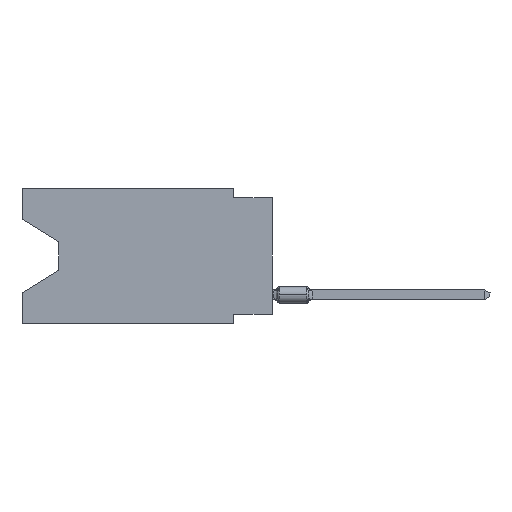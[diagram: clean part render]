
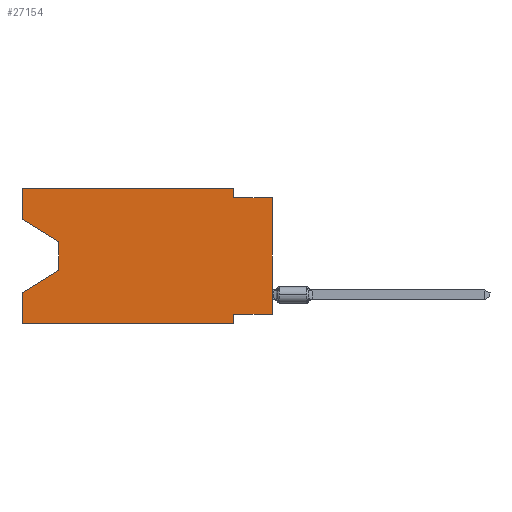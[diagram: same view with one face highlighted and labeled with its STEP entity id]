
A CAD part, left-side view. The second image highlights one B-rep face of the part: STEP entity #27154.
In plain terms, the highlighted planar face has unit normal (-1, 0, 0).
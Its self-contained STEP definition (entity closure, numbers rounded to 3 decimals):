
#526 = CARTESIAN_POINT ( 'NONE',  ( 0., 13.97, -3.505 ) ) ;
#664 = DIRECTION ( 'NONE',  ( 0., -1., 0. ) ) ;
#1069 = ORIENTED_EDGE ( 'NONE', *, *, #26090, .F. ) ;
#1391 = EDGE_LOOP ( 'NONE', ( #17667, #36850, #2581, #44364, #42576, #38319, #42074, #20796, #1069, #49209, #34071, #36737 ) ) ;
#1396 = VERTEX_POINT ( 'NONE', #10982 ) ;
#2026 = VECTOR ( 'NONE', #36965, 1000. ) ;
#2171 = EDGE_CURVE ( 'NONE', #13277, #44504, #7679, .T. ) ;
#2351 = VERTEX_POINT ( 'NONE', #28143 ) ;
#2581 = ORIENTED_EDGE ( 'NONE', *, *, #29722, .T. ) ;
#3048 = VECTOR ( 'NONE', #36815, 1000. ) ;
#4729 = VECTOR ( 'NONE', #34349, 1000. ) ;
#4867 = VECTOR ( 'NONE', #17695, 1000. ) ;
#5331 = EDGE_CURVE ( 'NONE', #1396, #10738, #50507, .T. ) ;
#6120 = CARTESIAN_POINT ( 'NONE',  ( 0., 13.97, -5.385 ) ) ;
#7053 = EDGE_CURVE ( 'NONE', #44504, #2351, #36006, .T. ) ;
#7087 = DIRECTION ( 'NONE',  ( 0., 0., -1. ) ) ;
#7679 = LINE ( 'NONE', #27627, #4729 ) ;
#8245 = LINE ( 'NONE', #28692, #2026 ) ;
#8286 = EDGE_CURVE ( 'NONE', #1396, #45997, #10141, .T. ) ;
#9231 = VECTOR ( 'NONE', #21283, 1000. ) ;
#9792 = AXIS2_PLACEMENT_3D ( 'NONE', #19267, #10950, #31141 ) ;
#10141 = LINE ( 'NONE', #45111, #4867 ) ;
#10183 = DIRECTION ( 'NONE',  ( 0., 0., 1. ) ) ;
#10738 = VERTEX_POINT ( 'NONE', #27488 ) ;
#10950 = DIRECTION ( 'NONE',  ( 1., 0., 0. ) ) ;
#10982 = CARTESIAN_POINT ( 'NONE',  ( 0., 0., -8.255 ) ) ;
#11155 = VECTOR ( 'NONE', #664, 1000. ) ;
#12522 = CARTESIAN_POINT ( 'NONE',  ( 0., 2.54, -8.89 ) ) ;
#13277 = VERTEX_POINT ( 'NONE', #42623 ) ;
#13744 = VERTEX_POINT ( 'NONE', #28295 ) ;
#14079 = VERTEX_POINT ( 'NONE', #526 ) ;
#14117 = CARTESIAN_POINT ( 'NONE',  ( 0., 16.383, -2.038 ) ) ;
#14336 = LINE ( 'NONE', #34513, #37570 ) ;
#14949 = VECTOR ( 'NONE', #44714, 1000. ) ;
#14989 = EDGE_CURVE ( 'NONE', #13277, #14079, #45178, .T. ) ;
#16276 = CARTESIAN_POINT ( 'NONE',  ( 0., 13.97, -5.385 ) ) ;
#16737 = EDGE_CURVE ( 'NONE', #2351, #28925, #19806, .T. ) ;
#17667 = ORIENTED_EDGE ( 'NONE', *, *, #14989, .T. ) ;
#17695 = DIRECTION ( 'NONE',  ( 0., 1., 0. ) ) ;
#19267 = CARTESIAN_POINT ( 'NONE',  ( 0., 16.383, 0. ) ) ;
#19806 = LINE ( 'NONE', #35804, #40992 ) ;
#20115 = CARTESIAN_POINT ( 'NONE',  ( 0., 16.383, -8.89 ) ) ;
#20515 = VERTEX_POINT ( 'NONE', #6120 ) ;
#20796 = ORIENTED_EDGE ( 'NONE', *, *, #5331, .T. ) ;
#21283 = DIRECTION ( 'NONE',  ( 0., -1., 0. ) ) ;
#22308 = EDGE_CURVE ( 'NONE', #13744, #24663, #43385, .T. ) ;
#23673 = DIRECTION ( 'NONE',  ( 0., 0., -1. ) ) ;
#24663 = VERTEX_POINT ( 'NONE', #12522 ) ;
#26090 = EDGE_CURVE ( 'NONE', #28925, #10738, #40700, .T. ) ;
#26498 = PLANE ( 'NONE',  #9792 ) ;
#27154 = ADVANCED_FACE ( 'NONE', ( #35022 ), #26498, .F. ) ;
#27488 = CARTESIAN_POINT ( 'NONE',  ( 0., 0., -0.635 ) ) ;
#27627 = CARTESIAN_POINT ( 'NONE',  ( 0., 16.383, 0. ) ) ;
#28143 = CARTESIAN_POINT ( 'NONE',  ( 0., 2.54, 0. ) ) ;
#28295 = CARTESIAN_POINT ( 'NONE',  ( 0., 16.383, -8.89 ) ) ;
#28692 = CARTESIAN_POINT ( 'NONE',  ( 0., 2.54, -8.89 ) ) ;
#28896 = DIRECTION ( 'NONE',  ( 0., -0.855, -0.519 ) ) ;
#28925 = VERTEX_POINT ( 'NONE', #33757 ) ;
#28927 = LINE ( 'NONE', #16276, #14949 ) ;
#29060 = CARTESIAN_POINT ( 'NONE',  ( 0., 0., -0.635 ) ) ;
#29722 = EDGE_CURVE ( 'NONE', #20515, #32320, #28927, .T. ) ;
#30378 = CARTESIAN_POINT ( 'NONE',  ( 0., 2.54, -8.255 ) ) ;
#30651 = LINE ( 'NONE', #42552, #49188 ) ;
#31141 = DIRECTION ( 'NONE',  ( 0., 0., -1. ) ) ;
#32320 = VERTEX_POINT ( 'NONE', #46088 ) ;
#33757 = CARTESIAN_POINT ( 'NONE',  ( 0., 2.54, -0.635 ) ) ;
#34011 = CARTESIAN_POINT ( 'NONE',  ( 0., 16.383, 0. ) ) ;
#34071 = ORIENTED_EDGE ( 'NONE', *, *, #7053, .F. ) ;
#34349 = DIRECTION ( 'NONE',  ( 0., 0., 1. ) ) ;
#34513 = CARTESIAN_POINT ( 'NONE',  ( 0., 16.383, 0. ) ) ;
#35022 = FACE_OUTER_BOUND ( 'NONE', #1391, .T. ) ;
#35225 = DIRECTION ( 'NONE',  ( 0., 0., 1. ) ) ;
#35804 = CARTESIAN_POINT ( 'NONE',  ( 0., 2.54, 0. ) ) ;
#36006 = LINE ( 'NONE', #36526, #9231 ) ;
#36526 = CARTESIAN_POINT ( 'NONE',  ( 0., 16.383, 0. ) ) ;
#36737 = ORIENTED_EDGE ( 'NONE', *, *, #2171, .F. ) ;
#36815 = DIRECTION ( 'NONE',  ( 0., -1., 0. ) ) ;
#36850 = ORIENTED_EDGE ( 'NONE', *, *, #41946, .T. ) ;
#36965 = DIRECTION ( 'NONE',  ( 0., 0., -1. ) ) ;
#37570 = VECTOR ( 'NONE', #10183, 1000. ) ;
#38105 = VECTOR ( 'NONE', #35225, 1000. ) ;
#38319 = ORIENTED_EDGE ( 'NONE', *, *, #41251, .F. ) ;
#39367 = CARTESIAN_POINT ( 'NONE',  ( 0., 0., 0. ) ) ;
#40700 = LINE ( 'NONE', #29060, #3048 ) ;
#40992 = VECTOR ( 'NONE', #23673, 1000. ) ;
#41251 = EDGE_CURVE ( 'NONE', #45997, #24663, #8245, .T. ) ;
#41946 = EDGE_CURVE ( 'NONE', #14079, #20515, #30651, .T. ) ;
#42074 = ORIENTED_EDGE ( 'NONE', *, *, #8286, .F. ) ;
#42523 = VECTOR ( 'NONE', #28896, 1000. ) ;
#42552 = CARTESIAN_POINT ( 'NONE',  ( 0., 13.97, -3.505 ) ) ;
#42576 = ORIENTED_EDGE ( 'NONE', *, *, #22308, .T. ) ;
#42623 = CARTESIAN_POINT ( 'NONE',  ( 0., 16.383, -2.038 ) ) ;
#43182 = EDGE_CURVE ( 'NONE', #13744, #32320, #14336, .T. ) ;
#43385 = LINE ( 'NONE', #20115, #11155 ) ;
#44364 = ORIENTED_EDGE ( 'NONE', *, *, #43182, .F. ) ;
#44504 = VERTEX_POINT ( 'NONE', #34011 ) ;
#44714 = DIRECTION ( 'NONE',  ( 0., 0.855, -0.519 ) ) ;
#45111 = CARTESIAN_POINT ( 'NONE',  ( 0., 0., -8.255 ) ) ;
#45178 = LINE ( 'NONE', #14117, #42523 ) ;
#45997 = VERTEX_POINT ( 'NONE', #30378 ) ;
#46088 = CARTESIAN_POINT ( 'NONE',  ( 0., 16.383, -6.852 ) ) ;
#49188 = VECTOR ( 'NONE', #7087, 1000. ) ;
#49209 = ORIENTED_EDGE ( 'NONE', *, *, #16737, .F. ) ;
#50507 = LINE ( 'NONE', #39367, #38105 ) ;
